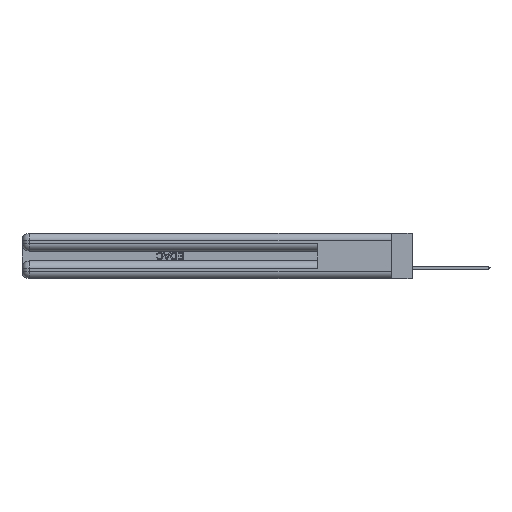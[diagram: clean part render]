
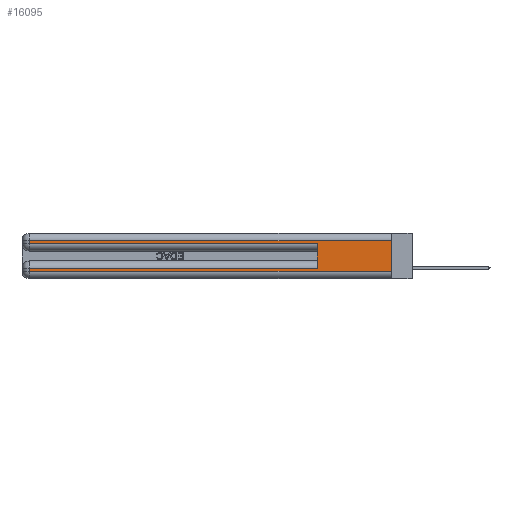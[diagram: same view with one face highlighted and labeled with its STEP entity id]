
A CAD part, left-side view. The second image highlights one B-rep face of the part: STEP entity #16095.
In plain terms, the highlighted planar face has unit normal (-1, 0, 0).
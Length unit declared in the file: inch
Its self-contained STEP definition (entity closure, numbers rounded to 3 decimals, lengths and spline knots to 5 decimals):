
#51 = VERTEX_POINT ( 'NONE', #50068 ) ;
#1387 = CARTESIAN_POINT ( 'NONE',  ( 0., 0.6, 0.085 ) ) ;
#2432 = ORIENTED_EDGE ( 'NONE', *, *, #4545, .T. ) ;
#2523 = DIRECTION ( 'NONE',  ( 0., 0., -1. ) ) ;
#3109 = EDGE_CURVE ( 'NONE', #12788, #37196, #39094, .T. ) ;
#3958 = VECTOR ( 'NONE', #2523, 39.37008 ) ;
#4027 = DIRECTION ( 'NONE',  ( 0., -1., 0. ) ) ;
#4456 = VECTOR ( 'NONE', #39258, 39.37008 ) ;
#4545 = EDGE_CURVE ( 'NONE', #37196, #30468, #13051, .T. ) ;
#6662 = VERTEX_POINT ( 'NONE', #49334 ) ;
#9188 = EDGE_CURVE ( 'NONE', #30468, #51, #36939, .T. ) ;
#9984 = CARTESIAN_POINT ( 'NONE',  ( 0., 0., 0.37 ) ) ;
#11729 = DIRECTION ( 'NONE',  ( 0., 1., 0. ) ) ;
#11994 = DIRECTION ( 'NONE',  ( 0., 0., -1. ) ) ;
#12676 = CARTESIAN_POINT ( 'NONE',  ( 0., 0.6, 0.145 ) ) ;
#12788 = VERTEX_POINT ( 'NONE', #45316 ) ;
#13008 = DIRECTION ( 'NONE',  ( 0., 0., 1. ) ) ;
#13051 = LINE ( 'NONE', #16381, #23709 ) ;
#13293 = EDGE_CURVE ( 'NONE', #6662, #38782, #50980, .T. ) ;
#14314 = CARTESIAN_POINT ( 'NONE',  ( 0., 0., 0.285 ) ) ;
#14971 = CARTESIAN_POINT ( 'NONE',  ( 0., 2.94, 0.06 ) ) ;
#16095 = ADVANCED_FACE ( 'NONE', ( #27629 ), #24045, .F. ) ;
#16281 = DIRECTION ( 'NONE',  ( 1., 0., 0. ) ) ;
#16312 = VERTEX_POINT ( 'NONE', #1387 ) ;
#16381 = CARTESIAN_POINT ( 'NONE',  ( 0., 2.94, 0.37 ) ) ;
#18348 = EDGE_CURVE ( 'NONE', #16312, #6662, #30003, .T. ) ;
#18719 = VECTOR ( 'NONE', #13008, 39.37008 ) ;
#19319 = EDGE_CURVE ( 'NONE', #16312, #51, #29979, .T. ) ;
#22531 = ORIENTED_EDGE ( 'NONE', *, *, #9188, .T. ) ;
#23709 = VECTOR ( 'NONE', #54197, 39.37008 ) ;
#24045 = PLANE ( 'NONE',  #50927 ) ;
#27277 = VERTEX_POINT ( 'NONE', #29802 ) ;
#27545 = CARTESIAN_POINT ( 'NONE',  ( 0., 2.94, 0.31 ) ) ;
#27629 = FACE_OUTER_BOUND ( 'NONE', #53588, .T. ) ;
#28055 = ORIENTED_EDGE ( 'NONE', *, *, #3109, .T. ) ;
#29105 = CARTESIAN_POINT ( 'NONE',  ( 0., 2.94, 0.285 ) ) ;
#29802 = CARTESIAN_POINT ( 'NONE',  ( 0., 0., 0.06 ) ) ;
#29979 = LINE ( 'NONE', #12676, #18719 ) ;
#30003 = LINE ( 'NONE', #32377, #34621 ) ;
#30468 = VERTEX_POINT ( 'NONE', #29105 ) ;
#30984 = ORIENTED_EDGE ( 'NONE', *, *, #19319, .F. ) ;
#32377 = CARTESIAN_POINT ( 'NONE',  ( 0., 0., 0.085 ) ) ;
#32390 = VECTOR ( 'NONE', #36829, 39.37008 ) ;
#33112 = LINE ( 'NONE', #35656, #32390 ) ;
#34273 = EDGE_CURVE ( 'NONE', #12788, #27277, #36249, .T. ) ;
#34621 = VECTOR ( 'NONE', #36662, 39.37008 ) ;
#35656 = CARTESIAN_POINT ( 'NONE',  ( 0., 0., 0.06 ) ) ;
#36249 = LINE ( 'NONE', #9984, #4456 ) ;
#36662 = DIRECTION ( 'NONE',  ( 0., 1., 0. ) ) ;
#36829 = DIRECTION ( 'NONE',  ( 0., -1., 0. ) ) ;
#36939 = LINE ( 'NONE', #14314, #38248 ) ;
#37196 = VERTEX_POINT ( 'NONE', #27545 ) ;
#37884 = ORIENTED_EDGE ( 'NONE', *, *, #42324, .T. ) ;
#38078 = ORIENTED_EDGE ( 'NONE', *, *, #34273, .F. ) ;
#38248 = VECTOR ( 'NONE', #4027, 39.37008 ) ;
#38782 = VERTEX_POINT ( 'NONE', #14971 ) ;
#39094 = LINE ( 'NONE', #53817, #49831 ) ;
#39258 = DIRECTION ( 'NONE',  ( 0., 0., -1. ) ) ;
#40074 = ORIENTED_EDGE ( 'NONE', *, *, #18348, .T. ) ;
#42324 = EDGE_CURVE ( 'NONE', #38782, #27277, #33112, .T. ) ;
#45316 = CARTESIAN_POINT ( 'NONE',  ( 0., 0., 0.31 ) ) ;
#49334 = CARTESIAN_POINT ( 'NONE',  ( 0., 2.94, 0.085 ) ) ;
#49831 = VECTOR ( 'NONE', #11729, 39.37008 ) ;
#50068 = CARTESIAN_POINT ( 'NONE',  ( 0., 0.6, 0.285 ) ) ;
#50927 = AXIS2_PLACEMENT_3D ( 'NONE', #53726, #16281, #11994 ) ;
#50980 = LINE ( 'NONE', #54122, #3958 ) ;
#53455 = ORIENTED_EDGE ( 'NONE', *, *, #13293, .T. ) ;
#53588 = EDGE_LOOP ( 'NONE', ( #38078, #28055, #2432, #22531, #30984, #40074, #53455, #37884 ) ) ;
#53726 = CARTESIAN_POINT ( 'NONE',  ( 0., 0., 0.37 ) ) ;
#53817 = CARTESIAN_POINT ( 'NONE',  ( 0., 0., 0.31 ) ) ;
#54122 = CARTESIAN_POINT ( 'NONE',  ( 0., 2.94, 0.37 ) ) ;
#54197 = DIRECTION ( 'NONE',  ( 0., 0., -1. ) ) ;
